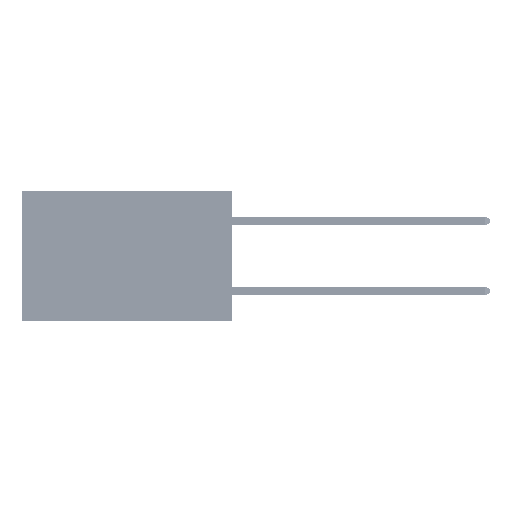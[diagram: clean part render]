
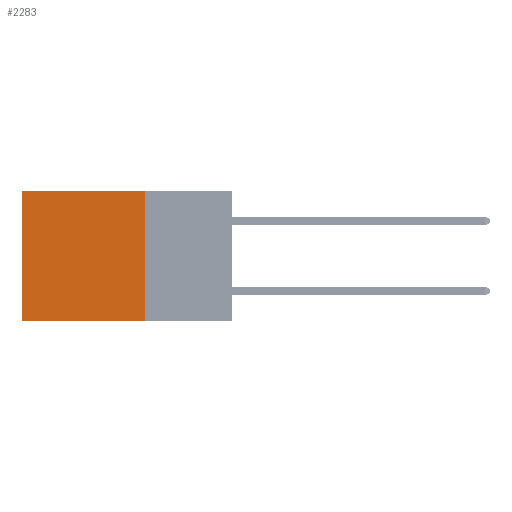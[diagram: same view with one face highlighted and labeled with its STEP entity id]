
A CAD part, left-side view. The second image highlights one B-rep face of the part: STEP entity #2283.
In plain terms, the highlighted planar face has unit normal (-1, 0, 0).
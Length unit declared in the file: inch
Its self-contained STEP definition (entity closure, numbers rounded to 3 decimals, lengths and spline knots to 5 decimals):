
#1518 = VERTEX_POINT ( 'NONE', #29581 ) ;
#2283 = ADVANCED_FACE ( 'NONE', ( #51203 ), #35048, .F. ) ;
#2936 = VECTOR ( 'NONE', #8007, 39.37008 ) ;
#3181 = EDGE_CURVE ( 'NONE', #18460, #1518, #31829, .T. ) ;
#3442 = ORIENTED_EDGE ( 'NONE', *, *, #40992, .F. ) ;
#7267 = LINE ( 'NONE', #51960, #17012 ) ;
#7282 = DIRECTION ( 'NONE',  ( 0., 0., -1. ) ) ;
#8007 = DIRECTION ( 'NONE',  ( 0., 1., 0. ) ) ;
#9951 = CARTESIAN_POINT ( 'NONE',  ( 0.2875, 0.25, 0. ) ) ;
#10963 = DIRECTION ( 'NONE',  ( 1., 0., 0. ) ) ;
#14451 = VERTEX_POINT ( 'NONE', #51399 ) ;
#16632 = LINE ( 'NONE', #37510, #20296 ) ;
#17012 = VECTOR ( 'NONE', #31873, 39.37008 ) ;
#18066 = VERTEX_POINT ( 'NONE', #45535 ) ;
#18460 = VERTEX_POINT ( 'NONE', #9951 ) ;
#20296 = VECTOR ( 'NONE', #44406, 39.37008 ) ;
#27629 = VECTOR ( 'NONE', #47794, 39.37008 ) ;
#29581 = CARTESIAN_POINT ( 'NONE',  ( 0.2875, 0.6, 0. ) ) ;
#30266 = EDGE_CURVE ( 'NONE', #14451, #18066, #7267, .T. ) ;
#31392 = LINE ( 'NONE', #50992, #27629 ) ;
#31750 = EDGE_LOOP ( 'NONE', ( #34354, #47912, #3442, #37136 ) ) ;
#31829 = LINE ( 'NONE', #36045, #2936 ) ;
#31873 = DIRECTION ( 'NONE',  ( 0., 1., 0. ) ) ;
#34354 = ORIENTED_EDGE ( 'NONE', *, *, #44766, .T. ) ;
#35048 = PLANE ( 'NONE',  #51860 ) ;
#36045 = CARTESIAN_POINT ( 'NONE',  ( 0.2875, 0.25, 0. ) ) ;
#37136 = ORIENTED_EDGE ( 'NONE', *, *, #3181, .T. ) ;
#37510 = CARTESIAN_POINT ( 'NONE',  ( 0.2875, 0.6, 0. ) ) ;
#40992 = EDGE_CURVE ( 'NONE', #18460, #14451, #31392, .T. ) ;
#43255 = CARTESIAN_POINT ( 'NONE',  ( 0.2875, 0.25, 0. ) ) ;
#44406 = DIRECTION ( 'NONE',  ( 0., 0., -1. ) ) ;
#44766 = EDGE_CURVE ( 'NONE', #1518, #18066, #16632, .T. ) ;
#45535 = CARTESIAN_POINT ( 'NONE',  ( 0.2875, 0.6, -0.37 ) ) ;
#47794 = DIRECTION ( 'NONE',  ( 0., 0., -1. ) ) ;
#47912 = ORIENTED_EDGE ( 'NONE', *, *, #30266, .F. ) ;
#50992 = CARTESIAN_POINT ( 'NONE',  ( 0.2875, 0.25, 0. ) ) ;
#51203 = FACE_OUTER_BOUND ( 'NONE', #31750, .T. ) ;
#51399 = CARTESIAN_POINT ( 'NONE',  ( 0.2875, 0.25, -0.37 ) ) ;
#51860 = AXIS2_PLACEMENT_3D ( 'NONE', #43255, #10963, #7282 ) ;
#51960 = CARTESIAN_POINT ( 'NONE',  ( 0.2875, 0.25, -0.37 ) ) ;
